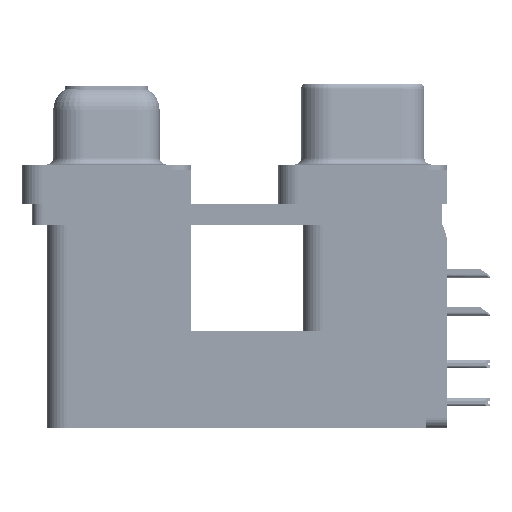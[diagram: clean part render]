
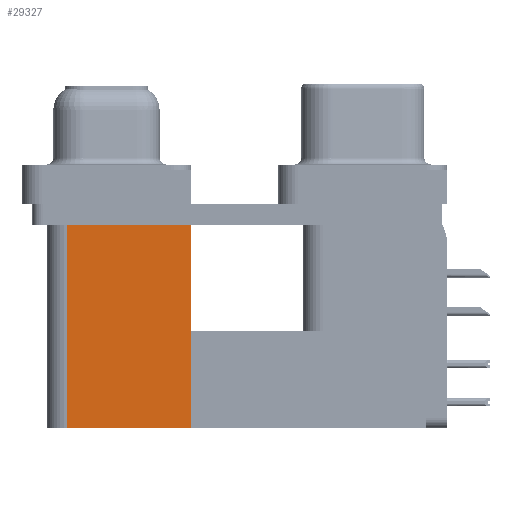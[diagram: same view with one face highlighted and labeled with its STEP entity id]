
A CAD part, left-side view. The second image highlights one B-rep face of the part: STEP entity #29327.
In plain terms, the highlighted planar face has unit normal (-1, 0, 0).
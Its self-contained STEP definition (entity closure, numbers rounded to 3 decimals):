
#2069 = VECTOR ( 'NONE', #2415, 1000. ) ;
#2180 = VECTOR ( 'NONE', #39696, 1000. ) ;
#2415 = DIRECTION ( 'NONE',  ( 0., 1., 0. ) ) ;
#4398 = CARTESIAN_POINT ( 'NONE',  ( 3.7, 12.775, -2.5 ) ) ;
#4453 = VERTEX_POINT ( 'NONE', #23086 ) ;
#4662 = DIRECTION ( 'NONE',  ( 0., 1., 0. ) ) ;
#5821 = CARTESIAN_POINT ( 'NONE',  ( 3.7, 21.975, -19.2 ) ) ;
#9798 = FACE_OUTER_BOUND ( 'NONE', #26522, .T. ) ;
#10341 = DIRECTION ( 'NONE',  ( 1., 0., 0. ) ) ;
#10619 = PLANE ( 'NONE',  #33717 ) ;
#14531 = EDGE_CURVE ( 'NONE', #41999, #53337, #42695, .T. ) ;
#18124 = DIRECTION ( 'NONE',  ( 0., 0., -1. ) ) ;
#23077 = ORIENTED_EDGE ( 'NONE', *, *, #44532, .F. ) ;
#23086 = CARTESIAN_POINT ( 'NONE',  ( 3.7, 12.775, -19.2 ) ) ;
#26522 = EDGE_LOOP ( 'NONE', ( #53610, #53483, #23077, #43005 ) ) ;
#27392 = CARTESIAN_POINT ( 'NONE',  ( 3.7, 12.775, -2.5 ) ) ;
#27637 = CARTESIAN_POINT ( 'NONE',  ( 3.7, 21.975, -2.5 ) ) ;
#27654 = LINE ( 'NONE', #48510, #2069 ) ;
#28064 = DIRECTION ( 'NONE',  ( 0., 0., 1. ) ) ;
#28559 = VECTOR ( 'NONE', #4662, 1000. ) ;
#29327 = ADVANCED_FACE ( 'NONE', ( #9798 ), #10619, .F. ) ;
#31342 = VERTEX_POINT ( 'NONE', #47433 ) ;
#32226 = CARTESIAN_POINT ( 'NONE',  ( 3.7, 12.775, -19.2 ) ) ;
#33717 = AXIS2_PLACEMENT_3D ( 'NONE', #39501, #10341, #18124 ) ;
#39419 = LINE ( 'NONE', #5821, #2180 ) ;
#39501 = CARTESIAN_POINT ( 'NONE',  ( 3.7, 12.775, -19.2 ) ) ;
#39696 = DIRECTION ( 'NONE',  ( 0., 0., 1. ) ) ;
#41310 = EDGE_CURVE ( 'NONE', #4453, #41999, #49185, .T. ) ;
#41999 = VERTEX_POINT ( 'NONE', #27392 ) ;
#42695 = LINE ( 'NONE', #4398, #28559 ) ;
#43005 = ORIENTED_EDGE ( 'NONE', *, *, #41310, .T. ) ;
#44532 = EDGE_CURVE ( 'NONE', #4453, #31342, #27654, .T. ) ;
#45272 = VECTOR ( 'NONE', #28064, 1000. ) ;
#47433 = CARTESIAN_POINT ( 'NONE',  ( 3.7, 21.975, -19.2 ) ) ;
#48510 = CARTESIAN_POINT ( 'NONE',  ( 3.7, 12.775, -19.2 ) ) ;
#49185 = LINE ( 'NONE', #32226, #45272 ) ;
#52767 = EDGE_CURVE ( 'NONE', #31342, #53337, #39419, .T. ) ;
#53337 = VERTEX_POINT ( 'NONE', #27637 ) ;
#53483 = ORIENTED_EDGE ( 'NONE', *, *, #52767, .F. ) ;
#53610 = ORIENTED_EDGE ( 'NONE', *, *, #14531, .T. ) ;
